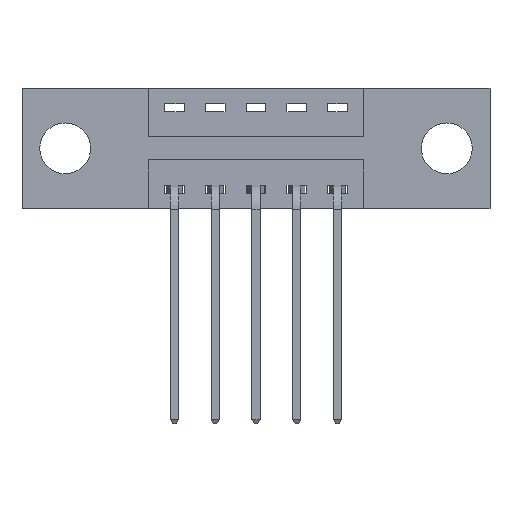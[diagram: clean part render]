
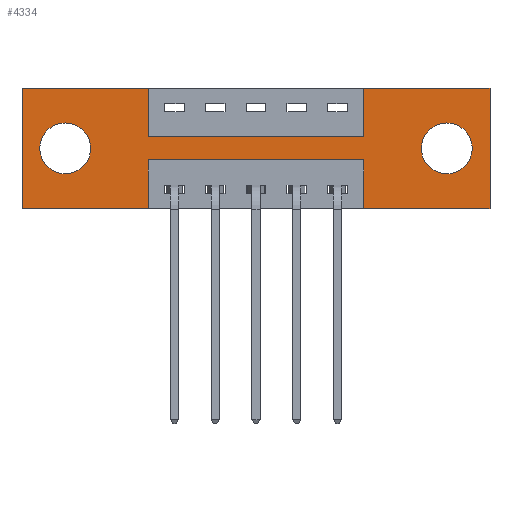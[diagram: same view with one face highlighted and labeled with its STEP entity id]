
A CAD part, front view. The second image highlights one B-rep face of the part: STEP entity #4334.
In plain terms, the highlighted planar face has unit normal (0, -1, 0).
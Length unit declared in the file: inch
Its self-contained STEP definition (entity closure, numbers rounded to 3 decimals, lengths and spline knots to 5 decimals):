
#10 = CARTESIAN_POINT ( 'NONE',  ( 0., 0., -0.37 ) ) ;
#23 = VECTOR ( 'NONE', #7178, 39.37008 ) ;
#38 = EDGE_LOOP ( 'NONE', ( #1669, #1004 ) ) ;
#88 = LINE ( 'NONE', #7050, #8091 ) ;
#190 = EDGE_CURVE ( 'NONE', #6679, #1385, #3796, .T. ) ;
#250 = LINE ( 'NONE', #4760, #23 ) ;
#291 = VERTEX_POINT ( 'NONE', #1082 ) ;
#315 = CARTESIAN_POINT ( 'NONE',  ( 1.435, 0., 0. ) ) ;
#561 = CARTESIAN_POINT ( 'NONE',  ( 1.0475, 0., -0.15 ) ) ;
#620 = DIRECTION ( 'NONE',  ( 0., 0., -1. ) ) ;
#660 = ORIENTED_EDGE ( 'NONE', *, *, #2953, .F. ) ;
#663 = DIRECTION ( 'NONE',  ( 0., 0., 1. ) ) ;
#699 = CARTESIAN_POINT ( 'NONE',  ( 1.435, 0., 0. ) ) ;
#705 = ORIENTED_EDGE ( 'NONE', *, *, #3470, .F. ) ;
#707 = AXIS2_PLACEMENT_3D ( 'NONE', #3309, #7561, #3938 ) ;
#719 = DIRECTION ( 'NONE',  ( 0., 0., -1. ) ) ;
#902 = EDGE_CURVE ( 'NONE', #6307, #3714, #3788, .T. ) ;
#967 = CARTESIAN_POINT ( 'NONE',  ( 0., 0., 0. ) ) ;
#1004 = ORIENTED_EDGE ( 'NONE', *, *, #5113, .T. ) ;
#1053 = EDGE_CURVE ( 'NONE', #291, #1584, #4868, .T. ) ;
#1076 = CARTESIAN_POINT ( 'NONE',  ( 0., 0., -0.37 ) ) ;
#1082 = CARTESIAN_POINT ( 'NONE',  ( 0.1325, 0., -0.263 ) ) ;
#1169 = EDGE_CURVE ( 'NONE', #1584, #291, #4272, .T. ) ;
#1192 = VECTOR ( 'NONE', #5952, 39.37008 ) ;
#1261 = VERTEX_POINT ( 'NONE', #7679 ) ;
#1325 = DIRECTION ( 'NONE',  ( 0., 0., 1. ) ) ;
#1331 = ORIENTED_EDGE ( 'NONE', *, *, #1169, .T. ) ;
#1385 = VERTEX_POINT ( 'NONE', #7753 ) ;
#1435 = CARTESIAN_POINT ( 'NONE',  ( 0.1325, 0., -0.185 ) ) ;
#1555 = ORIENTED_EDGE ( 'NONE', *, *, #1053, .T. ) ;
#1584 = VERTEX_POINT ( 'NONE', #6616 ) ;
#1617 = ORIENTED_EDGE ( 'NONE', *, *, #2432, .F. ) ;
#1669 = ORIENTED_EDGE ( 'NONE', *, *, #8021, .T. ) ;
#1787 = CARTESIAN_POINT ( 'NONE',  ( 0.3875, 0., -0.22 ) ) ;
#1799 = AXIS2_PLACEMENT_3D ( 'NONE', #1435, #6560, #3926 ) ;
#1807 = ORIENTED_EDGE ( 'NONE', *, *, #1990, .F. ) ;
#1855 = DIRECTION ( 'NONE',  ( 1., 0., 0. ) ) ;
#1952 = ORIENTED_EDGE ( 'NONE', *, *, #7452, .F. ) ;
#1953 = DIRECTION ( 'NONE',  ( 0., 0., 1. ) ) ;
#1990 = EDGE_CURVE ( 'NONE', #3459, #6370, #4145, .T. ) ;
#2077 = CIRCLE ( 'NONE', #4151, 0.078 ) ;
#2098 = ORIENTED_EDGE ( 'NONE', *, *, #7867, .F. ) ;
#2149 = VECTOR ( 'NONE', #3930, 39.37008 ) ;
#2154 = VECTOR ( 'NONE', #2502, 39.37008 ) ;
#2220 = AXIS2_PLACEMENT_3D ( 'NONE', #7660, #7770, #663 ) ;
#2432 = EDGE_CURVE ( 'NONE', #6138, #6307, #88, .T. ) ;
#2474 = ORIENTED_EDGE ( 'NONE', *, *, #7010, .F. ) ;
#2502 = DIRECTION ( 'NONE',  ( 0., 0., -1. ) ) ;
#2527 = VECTOR ( 'NONE', #3717, 39.37008 ) ;
#2706 = ORIENTED_EDGE ( 'NONE', *, *, #5518, .F. ) ;
#2714 = PLANE ( 'NONE',  #707 ) ;
#2773 = DIRECTION ( 'NONE',  ( 1., 0., 0. ) ) ;
#2792 = LINE ( 'NONE', #5256, #5917 ) ;
#2845 = CARTESIAN_POINT ( 'NONE',  ( 1.3025, 0., -0.263 ) ) ;
#2921 = LINE ( 'NONE', #10, #1192 ) ;
#2935 = EDGE_LOOP ( 'NONE', ( #1807, #1952, #2098, #2474, #4612, #2706, #4028, #3566, #3478, #1617, #660, #705 ) ) ;
#2953 = EDGE_CURVE ( 'NONE', #5644, #6138, #6954, .T. ) ;
#3250 = DIRECTION ( 'NONE',  ( 1., 0., 0. ) ) ;
#3258 = CARTESIAN_POINT ( 'NONE',  ( 1.0475, 0., -0.22 ) ) ;
#3281 = VECTOR ( 'NONE', #3770, 39.37008 ) ;
#3309 = CARTESIAN_POINT ( 'NONE',  ( 0., 0., -0.37 ) ) ;
#3378 = AXIS2_PLACEMENT_3D ( 'NONE', #8164, #4601, #719 ) ;
#3459 = VERTEX_POINT ( 'NONE', #1787 ) ;
#3470 = EDGE_CURVE ( 'NONE', #6370, #5644, #6948, .T. ) ;
#3478 = ORIENTED_EDGE ( 'NONE', *, *, #902, .F. ) ;
#3566 = ORIENTED_EDGE ( 'NONE', *, *, #3937, .F. ) ;
#3714 = VERTEX_POINT ( 'NONE', #5714 ) ;
#3717 = DIRECTION ( 'NONE',  ( 0., 0., -1. ) ) ;
#3770 = DIRECTION ( 'NONE',  ( -1., 0., 0. ) ) ;
#3788 = LINE ( 'NONE', #7956, #2149 ) ;
#3796 = LINE ( 'NONE', #699, #2154 ) ;
#3799 = VECTOR ( 'NONE', #3250, 39.37008 ) ;
#3926 = DIRECTION ( 'NONE',  ( 0., 0., 1. ) ) ;
#3927 = VERTEX_POINT ( 'NONE', #8169 ) ;
#3930 = DIRECTION ( 'NONE',  ( 0., 0., -1. ) ) ;
#3937 = EDGE_CURVE ( 'NONE', #3714, #4699, #2792, .T. ) ;
#3938 = DIRECTION ( 'NONE',  ( 0., 0., -1. ) ) ;
#3991 = LINE ( 'NONE', #6972, #3799 ) ;
#4006 = CARTESIAN_POINT ( 'NONE',  ( 0., 0., -0.37 ) ) ;
#4015 = FACE_OUTER_BOUND ( 'NONE', #2935, .T. ) ;
#4028 = ORIENTED_EDGE ( 'NONE', *, *, #5739, .F. ) ;
#4145 = LINE ( 'NONE', #7157, #2527 ) ;
#4151 = AXIS2_PLACEMENT_3D ( 'NONE', #8095, #4527, #620 ) ;
#4257 = CARTESIAN_POINT ( 'NONE',  ( 1.0475, 0., -0.37 ) ) ;
#4272 = CIRCLE ( 'NONE', #2220, 0.078 ) ;
#4334 = ADVANCED_FACE ( 'NONE', ( #7443, #5706, #4015 ), #2714, .T. ) ;
#4426 = CARTESIAN_POINT ( 'NONE',  ( 0., 0., 0. ) ) ;
#4527 = DIRECTION ( 'NONE',  ( 0., 1., 0. ) ) ;
#4601 = DIRECTION ( 'NONE',  ( 0., 1., 0. ) ) ;
#4612 = ORIENTED_EDGE ( 'NONE', *, *, #190, .F. ) ;
#4699 = VERTEX_POINT ( 'NONE', #561 ) ;
#4760 = CARTESIAN_POINT ( 'NONE',  ( 1.0475, 0., 0. ) ) ;
#4768 = CIRCLE ( 'NONE', #3378, 0.078 ) ;
#4868 = CIRCLE ( 'NONE', #1799, 0.078 ) ;
#4924 = EDGE_LOOP ( 'NONE', ( #1331, #1555 ) ) ;
#5113 = EDGE_CURVE ( 'NONE', #5694, #1261, #2077, .T. ) ;
#5121 = VERTEX_POINT ( 'NONE', #3258 ) ;
#5180 = CARTESIAN_POINT ( 'NONE',  ( 0.3875, 0., -0.37 ) ) ;
#5256 = CARTESIAN_POINT ( 'NONE',  ( 0.3875, 0., -0.15 ) ) ;
#5331 = VECTOR ( 'NONE', #6164, 39.37008 ) ;
#5339 = VECTOR ( 'NONE', #1953, 39.37008 ) ;
#5518 = EDGE_CURVE ( 'NONE', #3927, #6679, #3991, .T. ) ;
#5643 = CARTESIAN_POINT ( 'NONE',  ( 0.3875, 0., -0.22 ) ) ;
#5644 = VERTEX_POINT ( 'NONE', #4006 ) ;
#5694 = VERTEX_POINT ( 'NONE', #2845 ) ;
#5706 = FACE_BOUND ( 'NONE', #4924, .T. ) ;
#5714 = CARTESIAN_POINT ( 'NONE',  ( 0.3875, 0., -0.15 ) ) ;
#5739 = EDGE_CURVE ( 'NONE', #4699, #3927, #250, .T. ) ;
#5758 = VECTOR ( 'NONE', #1325, 39.37008 ) ;
#5917 = VECTOR ( 'NONE', #2773, 39.37008 ) ;
#5952 = DIRECTION ( 'NONE',  ( -1., 0., 0. ) ) ;
#5959 = LINE ( 'NONE', #6385, #5758 ) ;
#6138 = VERTEX_POINT ( 'NONE', #967 ) ;
#6164 = DIRECTION ( 'NONE',  ( -1., 0., 0. ) ) ;
#6307 = VERTEX_POINT ( 'NONE', #8023 ) ;
#6370 = VERTEX_POINT ( 'NONE', #5180 ) ;
#6385 = CARTESIAN_POINT ( 'NONE',  ( 1.0475, 0., -0.37 ) ) ;
#6560 = DIRECTION ( 'NONE',  ( 0., 1., 0. ) ) ;
#6615 = LINE ( 'NONE', #5643, #3281 ) ;
#6616 = CARTESIAN_POINT ( 'NONE',  ( 0.1325, 0., -0.107 ) ) ;
#6679 = VERTEX_POINT ( 'NONE', #315 ) ;
#6948 = LINE ( 'NONE', #1076, #5331 ) ;
#6954 = LINE ( 'NONE', #4426, #5339 ) ;
#6972 = CARTESIAN_POINT ( 'NONE',  ( 0., 0., 0. ) ) ;
#7010 = EDGE_CURVE ( 'NONE', #1385, #7343, #2921, .T. ) ;
#7050 = CARTESIAN_POINT ( 'NONE',  ( 0., 0., 0. ) ) ;
#7157 = CARTESIAN_POINT ( 'NONE',  ( 0.3875, 0., -0.37 ) ) ;
#7178 = DIRECTION ( 'NONE',  ( 0., 0., 1. ) ) ;
#7343 = VERTEX_POINT ( 'NONE', #4257 ) ;
#7443 = FACE_BOUND ( 'NONE', #38, .T. ) ;
#7452 = EDGE_CURVE ( 'NONE', #5121, #3459, #6615, .T. ) ;
#7561 = DIRECTION ( 'NONE',  ( 0., -1., 0. ) ) ;
#7660 = CARTESIAN_POINT ( 'NONE',  ( 0.1325, 0., -0.185 ) ) ;
#7679 = CARTESIAN_POINT ( 'NONE',  ( 1.3025, 0., -0.107 ) ) ;
#7753 = CARTESIAN_POINT ( 'NONE',  ( 1.435, 0., -0.37 ) ) ;
#7770 = DIRECTION ( 'NONE',  ( 0., 1., 0. ) ) ;
#7867 = EDGE_CURVE ( 'NONE', #7343, #5121, #5959, .T. ) ;
#7956 = CARTESIAN_POINT ( 'NONE',  ( 0.3875, 0., 0. ) ) ;
#8021 = EDGE_CURVE ( 'NONE', #1261, #5694, #4768, .T. ) ;
#8023 = CARTESIAN_POINT ( 'NONE',  ( 0.3875, 0., 0. ) ) ;
#8091 = VECTOR ( 'NONE', #1855, 39.37008 ) ;
#8095 = CARTESIAN_POINT ( 'NONE',  ( 1.3025, 0., -0.185 ) ) ;
#8164 = CARTESIAN_POINT ( 'NONE',  ( 1.3025, 0., -0.185 ) ) ;
#8169 = CARTESIAN_POINT ( 'NONE',  ( 1.0475, 0., 0. ) ) ;
